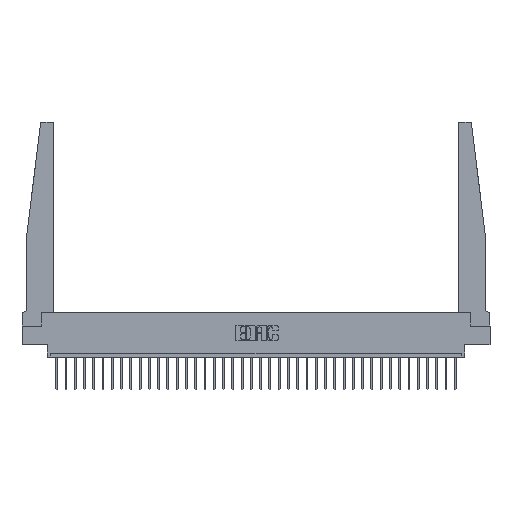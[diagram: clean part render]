
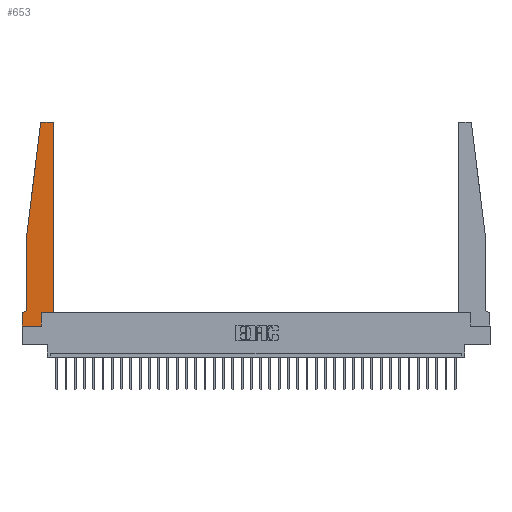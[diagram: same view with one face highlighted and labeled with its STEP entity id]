
A CAD part, top view. The second image highlights one B-rep face of the part: STEP entity #653.
In plain terms, the highlighted planar face has unit normal (0, 0, 1).
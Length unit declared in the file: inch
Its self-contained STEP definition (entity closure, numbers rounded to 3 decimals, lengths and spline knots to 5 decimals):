
#78 = CARTESIAN_POINT ( 'NONE',  ( 0.425, 0.18, 0.37 ) ) ;
#82 = LINE ( 'NONE', #1227, #25519 ) ;
#225 = CARTESIAN_POINT ( 'NONE',  ( 0.065, 1.25, 0.37 ) ) ;
#381 = EDGE_CURVE ( 'NONE', #4011, #19711, #10462, .T. ) ;
#395 = VERTEX_POINT ( 'NONE', #4638 ) ;
#653 = ADVANCED_FACE ( 'NONE', ( #1940 ), #18941, .T. ) ;
#751 = EDGE_CURVE ( 'NONE', #395, #12890, #25088, .T. ) ;
#1100 = AXIS2_PLACEMENT_3D ( 'NONE', #6199, #23400, #3933 ) ;
#1227 = CARTESIAN_POINT ( 'NONE',  ( 0.065, 1.25, 0.37 ) ) ;
#1472 = VECTOR ( 'NONE', #4518, 39.37008 ) ;
#1603 = ORIENTED_EDGE ( 'NONE', *, *, #16436, .T. ) ;
#1617 = ORIENTED_EDGE ( 'NONE', *, *, #14065, .T. ) ;
#1667 = CARTESIAN_POINT ( 'NONE',  ( 0.2605, 0.18, 0.37 ) ) ;
#1798 = EDGE_CURVE ( 'NONE', #30176, #1953, #27673, .T. ) ;
#1801 = VECTOR ( 'NONE', #20859, 39.37008 ) ;
#1883 = VERTEX_POINT ( 'NONE', #15007 ) ;
#1940 = FACE_OUTER_BOUND ( 'NONE', #6115, .T. ) ;
#1953 = VERTEX_POINT ( 'NONE', #225 ) ;
#2187 = DIRECTION ( 'NONE',  ( 1., 0., 0. ) ) ;
#2246 = ORIENTED_EDGE ( 'NONE', *, *, #9246, .T. ) ;
#2384 = ORIENTED_EDGE ( 'NONE', *, *, #12387, .T. ) ;
#3603 = CARTESIAN_POINT ( 'NONE',  ( 0., 0., 0.37 ) ) ;
#3933 = DIRECTION ( 'NONE',  ( 1., 0., 0. ) ) ;
#4011 = VERTEX_POINT ( 'NONE', #5536 ) ;
#4274 = CARTESIAN_POINT ( 'NONE',  ( 0., 0.1875, 0.37 ) ) ;
#4518 = DIRECTION ( 'NONE',  ( -1., 0., 0. ) ) ;
#4638 = CARTESIAN_POINT ( 'NONE',  ( 0., 0.1875, 0.37 ) ) ;
#5536 = CARTESIAN_POINT ( 'NONE',  ( 0.2605, 0., 0.37 ) ) ;
#5958 = VECTOR ( 'NONE', #17303, 39.37008 ) ;
#6115 = EDGE_LOOP ( 'NONE', ( #2246, #20648, #18392, #1603, #1617, #10486, #19437, #2384, #12341, #16754, #7917, #24131 ) ) ;
#6199 = CARTESIAN_POINT ( 'NONE',  ( 0.27653, 2.72, 0.37 ) ) ;
#6533 = DIRECTION ( 'NONE',  ( 0., -1., 0. ) ) ;
#7689 = AXIS2_PLACEMENT_3D ( 'NONE', #9411, #12080, #31470 ) ;
#7917 = ORIENTED_EDGE ( 'NONE', *, *, #22449, .T. ) ;
#7923 = VECTOR ( 'NONE', #16058, 39.37008 ) ;
#8354 = CARTESIAN_POINT ( 'NONE',  ( 0.015, 0.1875, 0.37 ) ) ;
#8542 = VECTOR ( 'NONE', #27436, 39.37008 ) ;
#9009 = CARTESIAN_POINT ( 'NONE',  ( 0.425, 0.18, 0.37 ) ) ;
#9246 = EDGE_CURVE ( 'NONE', #30099, #28303, #28386, .T. ) ;
#9411 = CARTESIAN_POINT ( 'NONE',  ( 0.015, 0.2375, 0.37 ) ) ;
#10462 = LINE ( 'NONE', #23347, #24325 ) ;
#10486 = ORIENTED_EDGE ( 'NONE', *, *, #19685, .T. ) ;
#10684 = DIRECTION ( 'NONE',  ( -0.122, -0.992, 0. ) ) ;
#10856 = VERTEX_POINT ( 'NONE', #9009 ) ;
#11089 = DIRECTION ( 'NONE',  ( 0., -1., 0. ) ) ;
#11792 = EDGE_CURVE ( 'NONE', #19711, #10856, #20960, .T. ) ;
#12080 = DIRECTION ( 'NONE',  ( 0., 0., -1. ) ) ;
#12341 = ORIENTED_EDGE ( 'NONE', *, *, #381, .T. ) ;
#12387 = EDGE_CURVE ( 'NONE', #12890, #4011, #12487, .T. ) ;
#12487 = LINE ( 'NONE', #27062, #5958 ) ;
#12890 = VERTEX_POINT ( 'NONE', #3603 ) ;
#13052 = VECTOR ( 'NONE', #10684, 39.37008 ) ;
#14065 = EDGE_CURVE ( 'NONE', #1883, #29071, #28905, .T. ) ;
#14912 = CARTESIAN_POINT ( 'NONE',  ( 0.425, 2.72, 0.37 ) ) ;
#14920 = CIRCLE ( 'NONE', #17674, 0.03 ) ;
#15007 = CARTESIAN_POINT ( 'NONE',  ( 0.065, 0.2375, 0.37 ) ) ;
#15835 = CARTESIAN_POINT ( 'NONE',  ( 0.425, 0.18, 0.37 ) ) ;
#16058 = DIRECTION ( 'NONE',  ( 1., 0., 0. ) ) ;
#16122 = EDGE_CURVE ( 'NONE', #28303, #30176, #16715, .T. ) ;
#16436 = EDGE_CURVE ( 'NONE', #1953, #1883, #82, .T. ) ;
#16715 = CIRCLE ( 'NONE', #1100, 0.03 ) ;
#16733 = DIRECTION ( 'NONE',  ( 0., 0., 1. ) ) ;
#16754 = ORIENTED_EDGE ( 'NONE', *, *, #11792, .T. ) ;
#17303 = DIRECTION ( 'NONE',  ( 1., 0., 0. ) ) ;
#17674 = AXIS2_PLACEMENT_3D ( 'NONE', #31508, #28999, #2187 ) ;
#18392 = ORIENTED_EDGE ( 'NONE', *, *, #1798, .T. ) ;
#18484 = DIRECTION ( 'NONE',  ( 0., 1., 0. ) ) ;
#18496 = VECTOR ( 'NONE', #11089, 39.37008 ) ;
#18941 = PLANE ( 'NONE',  #23807 ) ;
#19437 = ORIENTED_EDGE ( 'NONE', *, *, #751, .T. ) ;
#19685 = EDGE_CURVE ( 'NONE', #29071, #395, #26101, .T. ) ;
#19711 = VERTEX_POINT ( 'NONE', #1667 ) ;
#19898 = EDGE_CURVE ( 'NONE', #25210, #30099, #14920, .T. ) ;
#20648 = ORIENTED_EDGE ( 'NONE', *, *, #16122, .T. ) ;
#20651 = CARTESIAN_POINT ( 'NONE',  ( 0.25, 2.75, 0.37 ) ) ;
#20859 = DIRECTION ( 'NONE',  ( -1., 0., 0. ) ) ;
#20960 = LINE ( 'NONE', #15835, #7923 ) ;
#21014 = CARTESIAN_POINT ( 'NONE',  ( 0.27653, 2.75, 0.37 ) ) ;
#22449 = EDGE_CURVE ( 'NONE', #10856, #25210, #23155, .T. ) ;
#23155 = LINE ( 'NONE', #78, #8542 ) ;
#23347 = CARTESIAN_POINT ( 'NONE',  ( 0.2605, 0.18, 0.37 ) ) ;
#23400 = DIRECTION ( 'NONE',  ( 0., 0., 1. ) ) ;
#23807 = AXIS2_PLACEMENT_3D ( 'NONE', #4274, #16733, #23945 ) ;
#23945 = DIRECTION ( 'NONE',  ( 1., 0., 0. ) ) ;
#24131 = ORIENTED_EDGE ( 'NONE', *, *, #19898, .T. ) ;
#24325 = VECTOR ( 'NONE', #18484, 39.37008 ) ;
#24890 = CARTESIAN_POINT ( 'NONE',  ( 0.24675, 2.72367, 0.37 ) ) ;
#25088 = LINE ( 'NONE', #28419, #18496 ) ;
#25210 = VERTEX_POINT ( 'NONE', #14912 ) ;
#25395 = CARTESIAN_POINT ( 'NONE',  ( 0.065, 1.25, 0.37 ) ) ;
#25519 = VECTOR ( 'NONE', #6533, 39.37008 ) ;
#26101 = LINE ( 'NONE', #28711, #1472 ) ;
#27062 = CARTESIAN_POINT ( 'NONE',  ( 0., 0., 0.37 ) ) ;
#27436 = DIRECTION ( 'NONE',  ( 0., 1., 0. ) ) ;
#27673 = LINE ( 'NONE', #25395, #13052 ) ;
#28303 = VERTEX_POINT ( 'NONE', #21014 ) ;
#28386 = LINE ( 'NONE', #20651, #1801 ) ;
#28419 = CARTESIAN_POINT ( 'NONE',  ( 0., 0., 0.37 ) ) ;
#28711 = CARTESIAN_POINT ( 'NONE',  ( 0.065, 0.1875, 0.37 ) ) ;
#28905 = CIRCLE ( 'NONE', #7689, 0.05 ) ;
#28999 = DIRECTION ( 'NONE',  ( 0., 0., 1. ) ) ;
#29071 = VERTEX_POINT ( 'NONE', #8354 ) ;
#29399 = CARTESIAN_POINT ( 'NONE',  ( 0.395, 2.75, 0.37 ) ) ;
#30099 = VERTEX_POINT ( 'NONE', #29399 ) ;
#30176 = VERTEX_POINT ( 'NONE', #24890 ) ;
#31470 = DIRECTION ( 'NONE',  ( -1., 0., 0. ) ) ;
#31508 = CARTESIAN_POINT ( 'NONE',  ( 0.395, 2.72, 0.37 ) ) ;
